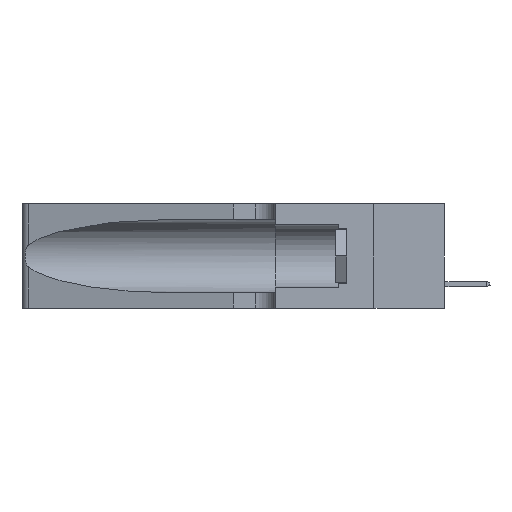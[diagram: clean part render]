
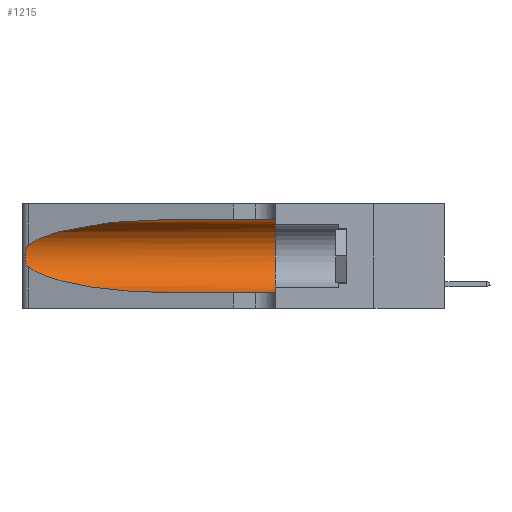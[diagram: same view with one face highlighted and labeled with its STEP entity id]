
A CAD part, left-side view. The second image highlights one B-rep face of the part: STEP entity #1215.
In plain terms, the highlighted cylindrical face has radius 3.308 mm (diameter 6.617 mm), a partial arc.
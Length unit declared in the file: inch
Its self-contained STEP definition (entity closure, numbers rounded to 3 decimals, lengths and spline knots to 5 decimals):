
#578 = AXIS2_PLACEMENT_3D ( 'NONE', #8210, #16958, #15396 ) ;
#592 = VECTOR ( 'NONE', #2890, 39.37008 ) ;
#728 = VECTOR ( 'NONE', #15359, 39.37008 ) ;
#1137 = CARTESIAN_POINT ( 'NONE',  ( 0.1305, 1.61858, 0.05475 ) ) ;
#1215 = ADVANCED_FACE ( 'NONE', ( #2095 ), #11684, .F. ) ;
#1761 = VERTEX_POINT ( 'NONE', #8117 ) ;
#1929 = CARTESIAN_POINT ( 'NONE',  ( 0.26018, 1.23835, 0.19895 ) ) ;
#2095 = FACE_OUTER_BOUND ( 'NONE', #7277, .T. ) ;
#2851 = EDGE_CURVE ( 'NONE', #11855, #14445, #9772, .T. ) ;
#2890 = DIRECTION ( 'NONE',  ( 0., -1., 0. ) ) ;
#2961 = CARTESIAN_POINT ( 'NONE',  ( 0.1305, 0.35, 0.31525 ) ) ;
#3054 = DIRECTION ( 'NONE',  ( 0., 1., 0. ) ) ;
#3072 = CARTESIAN_POINT ( 'NONE',  ( 0.25487, 1.22718, 0.14631 ) ) ;
#3343 = CARTESIAN_POINT ( 'NONE',  ( 0.26017, 1.23833, 0.17102 ) ) ;
#3573 = CARTESIAN_POINT ( 'NONE',  ( 0.1305, 0.35, 0.05475 ) ) ;
#3762 = CARTESIAN_POINT ( 'NONE',  ( 0.25555, 1.22993, 0.14849 ) ) ;
#3905 = EDGE_CURVE ( 'NONE', #17800, #8489, #17266, .T. ) ;
#4246 = CARTESIAN_POINT ( 'NONE',  ( 0.1305, 1.61858, 0.31525 ) ) ;
#4260 = CARTESIAN_POINT ( 'NONE',  ( 0.1305, 0.72297, 0.31525 ) ) ;
#4782 = CARTESIAN_POINT ( 'NONE',  ( 0.25856, 1.23593, 0.16098 ) ) ;
#4841 = CARTESIAN_POINT ( 'NONE',  ( 0.25789, 1.23486, 0.15765 ) ) ;
#4949 = CARTESIAN_POINT ( 'NONE',  ( 0.26075, 1.23896, 0.178 ) ) ;
#5637 = CARTESIAN_POINT ( 'NONE',  ( 0.2373, 1.15595, 0.08982 ) ) ;
#5963 = DIRECTION ( 'NONE',  ( 0., 0., 1. ) ) ;
#7277 = EDGE_LOOP ( 'NONE', ( #8035, #16859, #11313, #9227, #15519, #17508 ) ) ;
#7643 = CARTESIAN_POINT ( 'NONE',  ( 0.25487, 1.22718, 0.22369 ) ) ;
#7750 = CARTESIAN_POINT ( 'NONE',  ( 0.1305, 0.72297, 0.05475 ) ) ;
#8035 = ORIENTED_EDGE ( 'NONE', *, *, #11803, .T. ) ;
#8117 = CARTESIAN_POINT ( 'NONE',  ( 0.25487, 1.22718, 0.22369 ) ) ;
#8210 = CARTESIAN_POINT ( 'NONE',  ( 0.1305, 1.61858, 0.185 ) ) ;
#8221 = CIRCLE ( 'NONE', #12604, 0.13025 ) ;
#8226 = EDGE_CURVE ( 'NONE', #14445, #10765, #15835, .T. ) ;
#8489 = VERTEX_POINT ( 'NONE', #2961 ) ;
#9078 = CARTESIAN_POINT ( 'NONE',  ( 0.25555, 1.22994, 0.2215 ) ) ;
#9227 = ORIENTED_EDGE ( 'NONE', *, *, #8226, .T. ) ;
#9772 =( BOUNDED_CURVE ( )  B_SPLINE_CURVE ( 3, ( #14166, #5637, #15597, #10088 ),
 .UNSPECIFIED., .F., .F. ) 
 B_SPLINE_CURVE_WITH_KNOTS ( ( 4, 4 ),
 ( 3.44316, 4.71239 ),
 .UNSPECIFIED. ) 
 CURVE ( )  GEOMETRIC_REPRESENTATION_ITEM ( )  RATIONAL_B_SPLINE_CURVE ( ( 1., 0.87, 0.87, 1. ) ) 
 REPRESENTATION_ITEM ( '' )  );
#10014 = CARTESIAN_POINT ( 'NONE',  ( 0.1305, 0.72297, 0.31525 ) ) ;
#10088 = CARTESIAN_POINT ( 'NONE',  ( 0.1305, 0.72297, 0.05475 ) ) ;
#10476 = CARTESIAN_POINT ( 'NONE',  ( 0.25854, 1.2359, 0.20912 ) ) ;
#10765 = VERTEX_POINT ( 'NONE', #3573 ) ;
#11313 = ORIENTED_EDGE ( 'NONE', *, *, #2851, .T. ) ;
#11536 = CARTESIAN_POINT ( 'NONE',  ( 0.1305, 0.35, 0.185 ) ) ;
#11684 = CYLINDRICAL_SURFACE ( 'NONE', #578, 0.13025 ) ;
#11803 = EDGE_CURVE ( 'NONE', #17800, #1761, #12509, .T. ) ;
#11855 = VERTEX_POINT ( 'NONE', #3072 ) ;
#12070 = CARTESIAN_POINT ( 'NONE',  ( 0.25787, 1.23484, 0.2124 ) ) ;
#12509 =( BOUNDED_CURVE ( )  B_SPLINE_CURVE ( 3, ( #10014, #12791, #14218, #12850 ),
 .UNSPECIFIED., .F., .T. ) 
 B_SPLINE_CURVE_WITH_KNOTS ( ( 4, 4 ),
 ( 1.5708, 2.84003 ),
 .UNSPECIFIED. ) 
 CURVE ( )  GEOMETRIC_REPRESENTATION_ITEM ( )  RATIONAL_B_SPLINE_CURVE ( ( 1., 0.87, 0.87, 1. ) ) 
 REPRESENTATION_ITEM ( '' )  );
#12604 = AXIS2_PLACEMENT_3D ( 'NONE', #11536, #3054, #5963 ) ;
#12791 = CARTESIAN_POINT ( 'NONE',  ( 0.18966, 0.96281, 0.31525 ) ) ;
#12850 = CARTESIAN_POINT ( 'NONE',  ( 0.25487, 1.22718, 0.22369 ) ) ;
#13361 = EDGE_CURVE ( 'NONE', #8489, #10765, #8221, .T. ) ;
#13730 = CARTESIAN_POINT ( 'NONE',  ( 0.25639, 1.23186, 0.15144 ) ) ;
#14166 = CARTESIAN_POINT ( 'NONE',  ( 0.25487, 1.22718, 0.14631 ) ) ;
#14218 = CARTESIAN_POINT ( 'NONE',  ( 0.2373, 1.15595, 0.28018 ) ) ;
#14445 = VERTEX_POINT ( 'NONE', #7750 ) ;
#14450 = B_SPLINE_CURVE_WITH_KNOTS ( 'NONE', 3,
 ( #7643, #9078, #17835, #12070, #10476, #1929, #16347, #4949, #3343, #4782, #4841, #13730, #3762, #15021 ),
 .UNSPECIFIED., .F., .F.,
 ( 4, 2, 2, 2, 2, 2, 4 ),
 ( 0., 0.00027, 0.00053, 0.00107, 0.0016, 0.00187, 0.00214 ),
 .UNSPECIFIED. ) ;
#14750 = EDGE_CURVE ( 'NONE', #1761, #11855, #14450, .T. ) ;
#15021 = CARTESIAN_POINT ( 'NONE',  ( 0.25487, 1.22718, 0.14631 ) ) ;
#15359 = DIRECTION ( 'NONE',  ( 0., -1., 0. ) ) ;
#15396 = DIRECTION ( 'NONE',  ( 0., 0., -1. ) ) ;
#15519 = ORIENTED_EDGE ( 'NONE', *, *, #13361, .F. ) ;
#15597 = CARTESIAN_POINT ( 'NONE',  ( 0.18966, 0.96281, 0.05475 ) ) ;
#15835 = LINE ( 'NONE', #1137, #728 ) ;
#16347 = CARTESIAN_POINT ( 'NONE',  ( 0.26075, 1.23896, 0.19203 ) ) ;
#16859 = ORIENTED_EDGE ( 'NONE', *, *, #14750, .T. ) ;
#16958 = DIRECTION ( 'NONE',  ( 0., -1., 0. ) ) ;
#17266 = LINE ( 'NONE', #4246, #592 ) ;
#17508 = ORIENTED_EDGE ( 'NONE', *, *, #3905, .F. ) ;
#17800 = VERTEX_POINT ( 'NONE', #4260 ) ;
#17835 = CARTESIAN_POINT ( 'NONE',  ( 0.25639, 1.23184, 0.21858 ) ) ;
